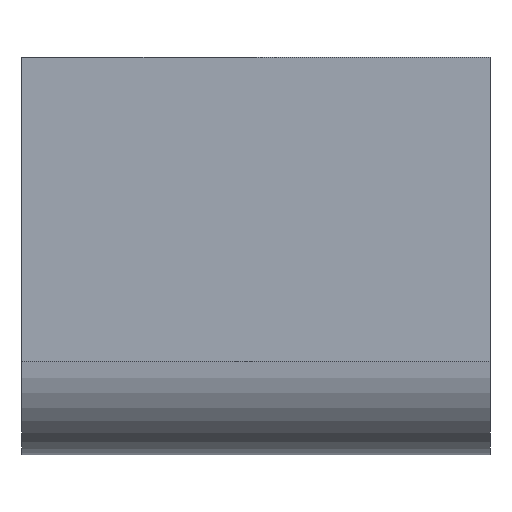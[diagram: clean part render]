
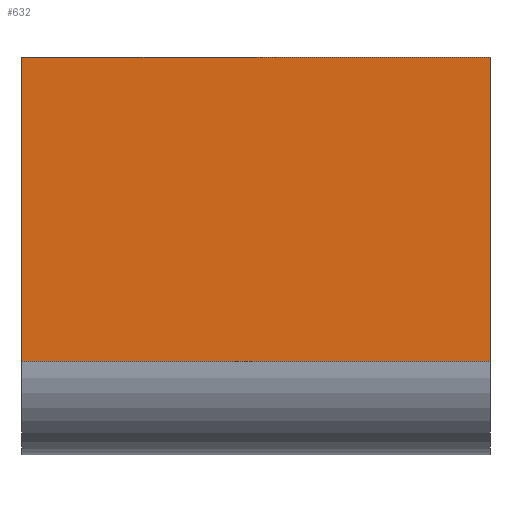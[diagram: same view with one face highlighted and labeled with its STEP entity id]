
A CAD part, front view. The second image highlights one B-rep face of the part: STEP entity #632.
In plain terms, the highlighted planar face has unit normal (0, -1, 0).
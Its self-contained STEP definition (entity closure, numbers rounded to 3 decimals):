
#8 = ORIENTED_EDGE ( 'NONE', *, *, #1836, .F. ) ;
#35 = ORIENTED_EDGE ( 'NONE', *, *, #520, .T. ) ;
#69 = VERTEX_POINT ( 'NONE', #1296 ) ;
#137 = LINE ( 'NONE', #1467, #222 ) ;
#215 = AXIS2_PLACEMENT_3D ( 'NONE', #551, #512, #506 ) ;
#222 = VECTOR ( 'NONE', #1462, 1000. ) ;
#226 = LINE ( 'NONE', #1306, #1092 ) ;
#228 = CARTESIAN_POINT ( 'NONE',  ( 50., -38.582, -58.094 ) ) ;
#234 = VERTEX_POINT ( 'NONE', #1480 ) ;
#262 = ORIENTED_EDGE ( 'NONE', *, *, #1015, .T. ) ;
#506 = DIRECTION ( 'NONE',  ( 0., 0., 1. ) ) ;
#512 = DIRECTION ( 'NONE',  ( 0., 1., 0. ) ) ;
#520 = EDGE_CURVE ( 'NONE', #69, #234, #137, .T. ) ;
#551 = CARTESIAN_POINT ( 'NONE',  ( 50., -38.582, -53.534 ) ) ;
#622 = CARTESIAN_POINT ( 'NONE',  ( 0., -38.582, -58.094 ) ) ;
#632 = ADVANCED_FACE ( 'NONE', ( #1548 ), #692, .F. ) ;
#692 = PLANE ( 'NONE',  #215 ) ;
#920 = VECTOR ( 'NONE', #1869, 1000. ) ;
#950 = LINE ( 'NONE', #1058, #920 ) ;
#1015 = EDGE_CURVE ( 'NONE', #234, #1666, #1451, .T. ) ;
#1023 = CARTESIAN_POINT ( 'NONE',  ( 0., -38.582, -53.534 ) ) ;
#1058 = CARTESIAN_POINT ( 'NONE',  ( 50., -38.582, -53.534 ) ) ;
#1092 = VECTOR ( 'NONE', #1315, 1000. ) ;
#1177 = DIRECTION ( 'NONE',  ( 0., 0., -1. ) ) ;
#1228 = EDGE_LOOP ( 'NONE', ( #262, #1903, #8, #35 ) ) ;
#1260 = VERTEX_POINT ( 'NONE', #228 ) ;
#1296 = CARTESIAN_POINT ( 'NONE',  ( 50., -38.582, -25.594 ) ) ;
#1306 = CARTESIAN_POINT ( 'NONE',  ( 50., -38.582, -58.094 ) ) ;
#1315 = DIRECTION ( 'NONE',  ( 1., 0., 0. ) ) ;
#1433 = VECTOR ( 'NONE', #1177, 1000. ) ;
#1451 = LINE ( 'NONE', #1023, #1433 ) ;
#1462 = DIRECTION ( 'NONE',  ( -1., 0., 0. ) ) ;
#1467 = CARTESIAN_POINT ( 'NONE',  ( 50., -38.582, -25.594 ) ) ;
#1480 = CARTESIAN_POINT ( 'NONE',  ( 0., -38.582, -25.594 ) ) ;
#1486 = EDGE_CURVE ( 'NONE', #1666, #1260, #226, .T. ) ;
#1548 = FACE_OUTER_BOUND ( 'NONE', #1228, .T. ) ;
#1666 = VERTEX_POINT ( 'NONE', #622 ) ;
#1836 = EDGE_CURVE ( 'NONE', #69, #1260, #950, .T. ) ;
#1869 = DIRECTION ( 'NONE',  ( 0., 0., -1. ) ) ;
#1903 = ORIENTED_EDGE ( 'NONE', *, *, #1486, .T. ) ;
